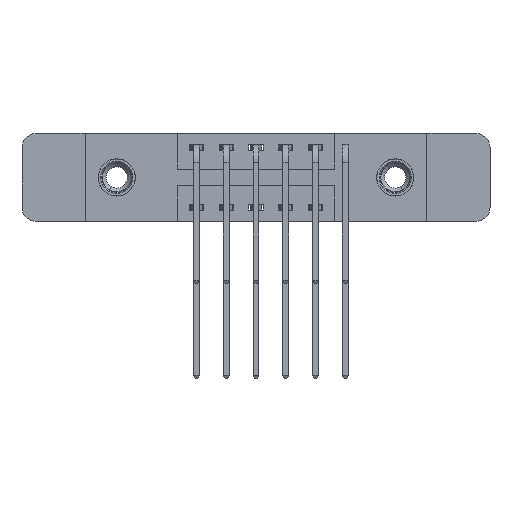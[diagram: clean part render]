
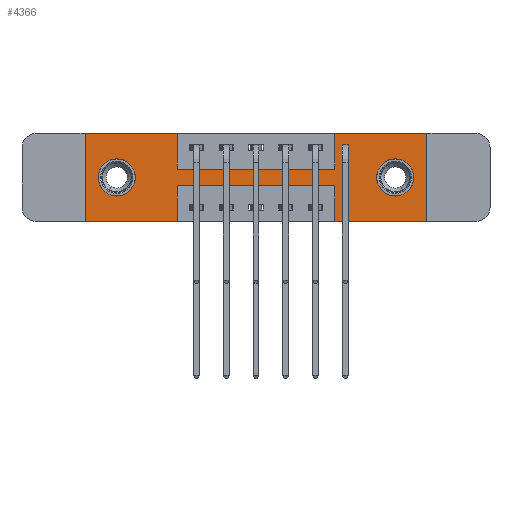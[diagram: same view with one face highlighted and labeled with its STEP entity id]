
A CAD part, front view. The second image highlights one B-rep face of the part: STEP entity #4366.
In plain terms, the highlighted planar face has unit normal (0, -1, 0).
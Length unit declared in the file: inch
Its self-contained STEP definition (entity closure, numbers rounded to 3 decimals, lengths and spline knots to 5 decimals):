
#362 = CARTESIAN_POINT ( 'NONE',  ( 0.1325, 0., -0.107 ) ) ;
#493 = CARTESIAN_POINT ( 'NONE',  ( 0.3875, 0., 0. ) ) ;
#650 = ORIENTED_EDGE ( 'NONE', *, *, #6098, .F. ) ;
#651 = LINE ( 'NONE', #493, #5613 ) ;
#708 = DIRECTION ( 'NONE',  ( 0., 1., 0. ) ) ;
#823 = EDGE_CURVE ( 'NONE', #3294, #9165, #651, .T. ) ;
#983 = VECTOR ( 'NONE', #9189, 39.37008 ) ;
#1031 = CARTESIAN_POINT ( 'NONE',  ( 0., 0., -0.37 ) ) ;
#1103 = DIRECTION ( 'NONE',  ( 1., 0., 0. ) ) ;
#1232 = EDGE_CURVE ( 'NONE', #1249, #4324, #15501, .T. ) ;
#1248 = EDGE_CURVE ( 'NONE', #15060, #8643, #7024, .T. ) ;
#1249 = VERTEX_POINT ( 'NONE', #10673 ) ;
#1437 = VERTEX_POINT ( 'NONE', #4777 ) ;
#1775 = ORIENTED_EDGE ( 'NONE', *, *, #10558, .T. ) ;
#1949 = EDGE_LOOP ( 'NONE', ( #5583, #12007 ) ) ;
#2354 = FACE_BOUND ( 'NONE', #6272, .T. ) ;
#2437 = FACE_BOUND ( 'NONE', #1949, .T. ) ;
#2577 = DIRECTION ( 'NONE',  ( 0., 0., -1. ) ) ;
#2657 = EDGE_CURVE ( 'NONE', #9165, #9106, #12009, .T. ) ;
#3201 = VERTEX_POINT ( 'NONE', #4219 ) ;
#3218 = CARTESIAN_POINT ( 'NONE',  ( 0.3875, 0., -0.37 ) ) ;
#3294 = VERTEX_POINT ( 'NONE', #11590 ) ;
#3328 = LINE ( 'NONE', #8173, #12366 ) ;
#3426 = CARTESIAN_POINT ( 'NONE',  ( 0., 0., -0.37 ) ) ;
#3488 = AXIS2_PLACEMENT_3D ( 'NONE', #15216, #14044, #15449 ) ;
#3637 = CARTESIAN_POINT ( 'NONE',  ( 1.3025, 0., -0.185 ) ) ;
#3949 = CARTESIAN_POINT ( 'NONE',  ( 1.0475, 0., -0.37 ) ) ;
#4219 = CARTESIAN_POINT ( 'NONE',  ( 1.0475, 0., -0.22 ) ) ;
#4295 = CARTESIAN_POINT ( 'NONE',  ( 0., 0., 0. ) ) ;
#4324 = VERTEX_POINT ( 'NONE', #9242 ) ;
#4366 = ADVANCED_FACE ( 'NONE', ( #2354, #2437, #7002 ), #10647, .T. ) ;
#4423 = EDGE_CURVE ( 'NONE', #7549, #1437, #11906, .T. ) ;
#4719 = EDGE_CURVE ( 'NONE', #13834, #5634, #10338, .T. ) ;
#4738 = VECTOR ( 'NONE', #13630, 39.37008 ) ;
#4777 = CARTESIAN_POINT ( 'NONE',  ( 1.0475, 0., -0.37 ) ) ;
#4850 = AXIS2_PLACEMENT_3D ( 'NONE', #9417, #708, #8218 ) ;
#4904 = LINE ( 'NONE', #8573, #14237 ) ;
#4957 = EDGE_CURVE ( 'NONE', #1437, #3201, #9765, .T. ) ;
#5583 = ORIENTED_EDGE ( 'NONE', *, *, #4719, .T. ) ;
#5603 = CARTESIAN_POINT ( 'NONE',  ( 0., 0., -0.37 ) ) ;
#5607 = VERTEX_POINT ( 'NONE', #10650 ) ;
#5613 = VECTOR ( 'NONE', #12687, 39.37008 ) ;
#5634 = VERTEX_POINT ( 'NONE', #9473 ) ;
#5861 = ORIENTED_EDGE ( 'NONE', *, *, #11379, .F. ) ;
#6098 = EDGE_CURVE ( 'NONE', #3201, #15060, #3328, .T. ) ;
#6145 = CARTESIAN_POINT ( 'NONE',  ( 0.3875, 0., -0.15 ) ) ;
#6272 = EDGE_LOOP ( 'NONE', ( #1775, #8016 ) ) ;
#6321 = VERTEX_POINT ( 'NONE', #5603 ) ;
#6671 = AXIS2_PLACEMENT_3D ( 'NONE', #3637, #8476, #2577 ) ;
#6974 = DIRECTION ( 'NONE',  ( 1., 0., 0. ) ) ;
#7002 = FACE_OUTER_BOUND ( 'NONE', #13160, .T. ) ;
#7024 = LINE ( 'NONE', #3218, #11464 ) ;
#7242 = VECTOR ( 'NONE', #1103, 39.37008 ) ;
#7379 = CARTESIAN_POINT ( 'NONE',  ( 1.0475, 0., -0.15 ) ) ;
#7549 = VERTEX_POINT ( 'NONE', #10156 ) ;
#7914 = CARTESIAN_POINT ( 'NONE',  ( 1.0475, 0., 0. ) ) ;
#7965 = EDGE_CURVE ( 'NONE', #9106, #5607, #14953, .T. ) ;
#8016 = ORIENTED_EDGE ( 'NONE', *, *, #1232, .T. ) ;
#8173 = CARTESIAN_POINT ( 'NONE',  ( 0.3875, 0., -0.22 ) ) ;
#8190 = CARTESIAN_POINT ( 'NONE',  ( 0., 0., -0.37 ) ) ;
#8218 = DIRECTION ( 'NONE',  ( 0., 0., -1. ) ) ;
#8460 = EDGE_CURVE ( 'NONE', #9858, #7549, #13919, .T. ) ;
#8476 = DIRECTION ( 'NONE',  ( 0., 1., 0. ) ) ;
#8498 = DIRECTION ( 'NONE',  ( 0., 0., -1. ) ) ;
#8543 = ORIENTED_EDGE ( 'NONE', *, *, #8460, .F. ) ;
#8573 = CARTESIAN_POINT ( 'NONE',  ( 0., 0., 0. ) ) ;
#8643 = VERTEX_POINT ( 'NONE', #14758 ) ;
#8653 = DIRECTION ( 'NONE',  ( 0., 1., 0. ) ) ;
#8656 = DIRECTION ( 'NONE',  ( 1., 0., 0. ) ) ;
#8675 = AXIS2_PLACEMENT_3D ( 'NONE', #14504, #8653, #13324 ) ;
#8684 = CIRCLE ( 'NONE', #8675, 0.078 ) ;
#8913 = ORIENTED_EDGE ( 'NONE', *, *, #7965, .F. ) ;
#9100 = VECTOR ( 'NONE', #9698, 39.37008 ) ;
#9106 = VERTEX_POINT ( 'NONE', #7379 ) ;
#9156 = DIRECTION ( 'NONE',  ( 0., 0., 1. ) ) ;
#9165 = VERTEX_POINT ( 'NONE', #11177 ) ;
#9171 = CARTESIAN_POINT ( 'NONE',  ( 0., 0., 0. ) ) ;
#9189 = DIRECTION ( 'NONE',  ( 0., 0., 1. ) ) ;
#9242 = CARTESIAN_POINT ( 'NONE',  ( 1.3025, 0., -0.107 ) ) ;
#9334 = EDGE_CURVE ( 'NONE', #8643, #6321, #11788, .T. ) ;
#9417 = CARTESIAN_POINT ( 'NONE',  ( 1.3025, 0., -0.185 ) ) ;
#9473 = CARTESIAN_POINT ( 'NONE',  ( 0.1325, 0., -0.263 ) ) ;
#9538 = VERTEX_POINT ( 'NONE', #9171 ) ;
#9546 = DIRECTION ( 'NONE',  ( 0., -1., 0. ) ) ;
#9698 = DIRECTION ( 'NONE',  ( -1., 0., 0. ) ) ;
#9765 = LINE ( 'NONE', #3949, #4738 ) ;
#9858 = VERTEX_POINT ( 'NONE', #10972 ) ;
#9978 = EDGE_CURVE ( 'NONE', #6321, #9538, #10340, .T. ) ;
#10128 = ORIENTED_EDGE ( 'NONE', *, *, #823, .F. ) ;
#10156 = CARTESIAN_POINT ( 'NONE',  ( 1.435, 0., -0.37 ) ) ;
#10219 = EDGE_CURVE ( 'NONE', #5607, #9858, #4904, .T. ) ;
#10338 = CIRCLE ( 'NONE', #3488, 0.078 ) ;
#10340 = LINE ( 'NONE', #4295, #12211 ) ;
#10558 = EDGE_CURVE ( 'NONE', #4324, #1249, #13229, .T. ) ;
#10647 = PLANE ( 'NONE',  #10855 ) ;
#10650 = CARTESIAN_POINT ( 'NONE',  ( 1.0475, 0., 0. ) ) ;
#10673 = CARTESIAN_POINT ( 'NONE',  ( 1.3025, 0., -0.263 ) ) ;
#10678 = VECTOR ( 'NONE', #10679, 39.37008 ) ;
#10679 = DIRECTION ( 'NONE',  ( -1., 0., 0. ) ) ;
#10776 = ORIENTED_EDGE ( 'NONE', *, *, #1248, .F. ) ;
#10855 = AXIS2_PLACEMENT_3D ( 'NONE', #3426, #9546, #8498 ) ;
#10972 = CARTESIAN_POINT ( 'NONE',  ( 1.435, 0., 0. ) ) ;
#11177 = CARTESIAN_POINT ( 'NONE',  ( 0.3875, 0., -0.15 ) ) ;
#11379 = EDGE_CURVE ( 'NONE', #9538, #3294, #15290, .T. ) ;
#11464 = VECTOR ( 'NONE', #15343, 39.37008 ) ;
#11535 = DIRECTION ( 'NONE',  ( 0., 0., -1. ) ) ;
#11590 = CARTESIAN_POINT ( 'NONE',  ( 0.3875, 0., 0. ) ) ;
#11788 = LINE ( 'NONE', #1031, #10678 ) ;
#11906 = LINE ( 'NONE', #8190, #9100 ) ;
#11945 = ORIENTED_EDGE ( 'NONE', *, *, #10219, .F. ) ;
#12007 = ORIENTED_EDGE ( 'NONE', *, *, #12400, .T. ) ;
#12009 = LINE ( 'NONE', #6145, #7242 ) ;
#12017 = ORIENTED_EDGE ( 'NONE', *, *, #9978, .F. ) ;
#12211 = VECTOR ( 'NONE', #9156, 39.37008 ) ;
#12366 = VECTOR ( 'NONE', #13007, 39.37008 ) ;
#12400 = EDGE_CURVE ( 'NONE', #5634, #13834, #8684, .T. ) ;
#12649 = CARTESIAN_POINT ( 'NONE',  ( 1.435, 0., 0. ) ) ;
#12687 = DIRECTION ( 'NONE',  ( 0., 0., -1. ) ) ;
#13007 = DIRECTION ( 'NONE',  ( -1., 0., 0. ) ) ;
#13160 = EDGE_LOOP ( 'NONE', ( #10776, #650, #13896, #13593, #8543, #11945, #8913, #13988, #10128, #5861, #12017, #14117 ) ) ;
#13229 = CIRCLE ( 'NONE', #6671, 0.078 ) ;
#13324 = DIRECTION ( 'NONE',  ( 0., 0., 1. ) ) ;
#13463 = CARTESIAN_POINT ( 'NONE',  ( 0.3875, 0., -0.22 ) ) ;
#13593 = ORIENTED_EDGE ( 'NONE', *, *, #4423, .F. ) ;
#13630 = DIRECTION ( 'NONE',  ( 0., 0., 1. ) ) ;
#13834 = VERTEX_POINT ( 'NONE', #362 ) ;
#13896 = ORIENTED_EDGE ( 'NONE', *, *, #4957, .F. ) ;
#13919 = LINE ( 'NONE', #12649, #14440 ) ;
#13988 = ORIENTED_EDGE ( 'NONE', *, *, #2657, .F. ) ;
#14044 = DIRECTION ( 'NONE',  ( 0., 1., 0. ) ) ;
#14117 = ORIENTED_EDGE ( 'NONE', *, *, #9334, .F. ) ;
#14237 = VECTOR ( 'NONE', #8656, 39.37008 ) ;
#14440 = VECTOR ( 'NONE', #11535, 39.37008 ) ;
#14456 = VECTOR ( 'NONE', #6974, 39.37008 ) ;
#14504 = CARTESIAN_POINT ( 'NONE',  ( 0.1325, 0., -0.185 ) ) ;
#14758 = CARTESIAN_POINT ( 'NONE',  ( 0.3875, 0., -0.37 ) ) ;
#14953 = LINE ( 'NONE', #7914, #983 ) ;
#15060 = VERTEX_POINT ( 'NONE', #13463 ) ;
#15209 = CARTESIAN_POINT ( 'NONE',  ( 0., 0., 0. ) ) ;
#15216 = CARTESIAN_POINT ( 'NONE',  ( 0.1325, 0., -0.185 ) ) ;
#15290 = LINE ( 'NONE', #15209, #14456 ) ;
#15343 = DIRECTION ( 'NONE',  ( 0., 0., -1. ) ) ;
#15449 = DIRECTION ( 'NONE',  ( 0., 0., 1. ) ) ;
#15501 = CIRCLE ( 'NONE', #4850, 0.078 ) ;
